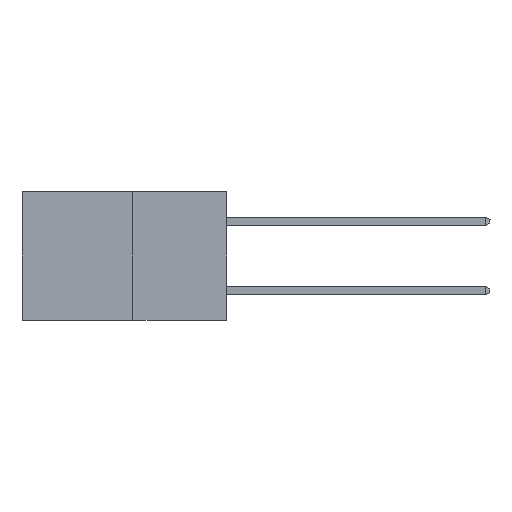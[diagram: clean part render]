
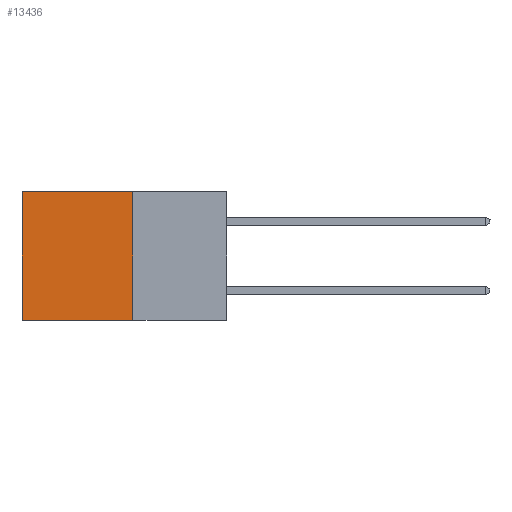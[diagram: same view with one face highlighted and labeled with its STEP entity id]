
A CAD part, left-side view. The second image highlights one B-rep face of the part: STEP entity #13436.
In plain terms, the highlighted planar face has unit normal (-1, 0, 0).
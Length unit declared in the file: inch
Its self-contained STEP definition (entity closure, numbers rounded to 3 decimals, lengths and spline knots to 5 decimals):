
#484 = CARTESIAN_POINT ( 'NONE',  ( 0.277, 0.59, -0.37 ) ) ;
#578 = VECTOR ( 'NONE', #9756, 39.37008 ) ;
#698 = CARTESIAN_POINT ( 'NONE',  ( 0.277, 0.27, -0.37 ) ) ;
#1356 = FACE_OUTER_BOUND ( 'NONE', #9705, .T. ) ;
#1461 = PLANE ( 'NONE',  #4250 ) ;
#1532 = CARTESIAN_POINT ( 'NONE',  ( 0.277, 0.27, -0.37 ) ) ;
#2055 = EDGE_CURVE ( 'NONE', #3619, #11690, #8213, .T. ) ;
#2077 = EDGE_CURVE ( 'NONE', #6564, #3619, #10752, .T. ) ;
#2270 = VECTOR ( 'NONE', #3190, 39.37008 ) ;
#2610 = DIRECTION ( 'NONE',  ( 1., 0., 0. ) ) ;
#2975 = EDGE_CURVE ( 'NONE', #4727, #11690, #8187, .T. ) ;
#3190 = DIRECTION ( 'NONE',  ( 0., 1., 0. ) ) ;
#3456 = ORIENTED_EDGE ( 'NONE', *, *, #2077, .T. ) ;
#3619 = VERTEX_POINT ( 'NONE', #9121 ) ;
#3901 = LINE ( 'NONE', #8741, #578 ) ;
#4250 = AXIS2_PLACEMENT_3D ( 'NONE', #5993, #2610, #10313 ) ;
#4699 = ORIENTED_EDGE ( 'NONE', *, *, #2055, .T. ) ;
#4727 = VERTEX_POINT ( 'NONE', #1532 ) ;
#4735 = CARTESIAN_POINT ( 'NONE',  ( 0.277, 0.27, 0. ) ) ;
#5316 = VECTOR ( 'NONE', #10505, 39.37008 ) ;
#5993 = CARTESIAN_POINT ( 'NONE',  ( 0.277, 0.27, -0.37 ) ) ;
#6119 = ORIENTED_EDGE ( 'NONE', *, *, #8662, .F. ) ;
#6564 = VERTEX_POINT ( 'NONE', #4735 ) ;
#6815 = CARTESIAN_POINT ( 'NONE',  ( 0.277, 0.27, 0. ) ) ;
#8187 = LINE ( 'NONE', #698, #11057 ) ;
#8213 = LINE ( 'NONE', #12453, #5316 ) ;
#8662 = EDGE_CURVE ( 'NONE', #6564, #4727, #3901, .T. ) ;
#8741 = CARTESIAN_POINT ( 'NONE',  ( 0.277, 0.27, -0.37 ) ) ;
#9121 = CARTESIAN_POINT ( 'NONE',  ( 0.277, 0.59, 0. ) ) ;
#9705 = EDGE_LOOP ( 'NONE', ( #4699, #10844, #6119, #3456 ) ) ;
#9756 = DIRECTION ( 'NONE',  ( 0., 0., -1. ) ) ;
#10313 = DIRECTION ( 'NONE',  ( 0., 0., -1. ) ) ;
#10505 = DIRECTION ( 'NONE',  ( 0., 0., -1. ) ) ;
#10616 = DIRECTION ( 'NONE',  ( 0., 1., 0. ) ) ;
#10752 = LINE ( 'NONE', #6815, #2270 ) ;
#10844 = ORIENTED_EDGE ( 'NONE', *, *, #2975, .F. ) ;
#11057 = VECTOR ( 'NONE', #10616, 39.37008 ) ;
#11690 = VERTEX_POINT ( 'NONE', #484 ) ;
#12453 = CARTESIAN_POINT ( 'NONE',  ( 0.277, 0.59, -0.37 ) ) ;
#13436 = ADVANCED_FACE ( 'NONE', ( #1356 ), #1461, .F. ) ;
